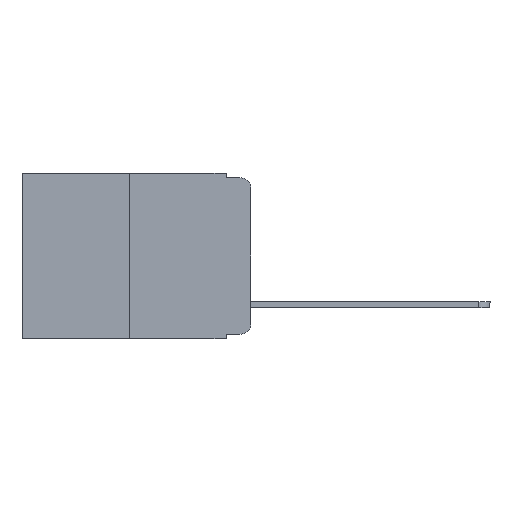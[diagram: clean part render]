
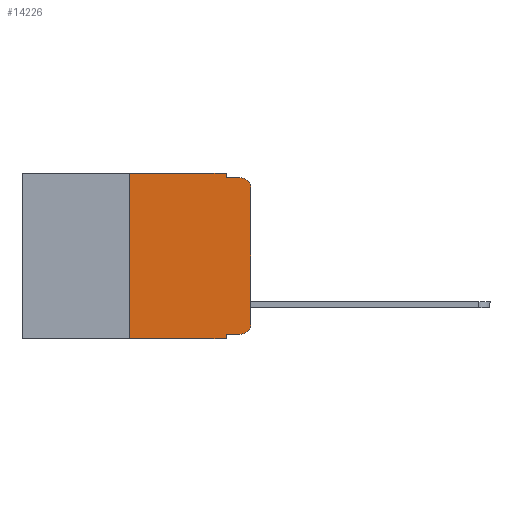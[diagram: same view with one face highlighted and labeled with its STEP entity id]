
A CAD part, left-side view. The second image highlights one B-rep face of the part: STEP entity #14226.
In plain terms, the highlighted planar face has unit normal (-1, 0, 0).
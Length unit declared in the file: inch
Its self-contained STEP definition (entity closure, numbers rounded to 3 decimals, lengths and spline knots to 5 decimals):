
#185 = DIRECTION ( 'NONE',  ( -1., 0., 0. ) ) ;
#280 = LINE ( 'NONE', #7466, #1851 ) ;
#344 = EDGE_CURVE ( 'NONE', #2409, #5183, #1535, .T. ) ;
#446 = VERTEX_POINT ( 'NONE', #1766 ) ;
#657 = DIRECTION ( 'NONE',  ( 0., -1., 0. ) ) ;
#705 = CARTESIAN_POINT ( 'NONE',  ( 0., 0.051, -0.01 ) ) ;
#978 = VECTOR ( 'NONE', #13768, 39.37008 ) ;
#1535 = LINE ( 'NONE', #14655, #6541 ) ;
#1602 = ORIENTED_EDGE ( 'NONE', *, *, #10612, .T. ) ;
#1671 = CARTESIAN_POINT ( 'NONE',  ( 0., 0., 0. ) ) ;
#1766 = CARTESIAN_POINT ( 'NONE',  ( 0., 0.25, -0.343 ) ) ;
#1851 = VECTOR ( 'NONE', #11121, 39.37008 ) ;
#1924 = DIRECTION ( 'NONE',  ( 0., 0., -1. ) ) ;
#1934 = VECTOR ( 'NONE', #12758, 39.37008 ) ;
#1949 = CARTESIAN_POINT ( 'NONE',  ( 0., 0., -0.03 ) ) ;
#2409 = VERTEX_POINT ( 'NONE', #8047 ) ;
#2477 = VECTOR ( 'NONE', #13080, 39.37008 ) ;
#2598 = CARTESIAN_POINT ( 'NONE',  ( 0., 0.02, -0.333 ) ) ;
#2870 = CARTESIAN_POINT ( 'NONE',  ( 0., 0.02, -0.01 ) ) ;
#3185 = ORIENTED_EDGE ( 'NONE', *, *, #9227, .F. ) ;
#3353 = LINE ( 'NONE', #7112, #5580 ) ;
#3398 = FACE_OUTER_BOUND ( 'NONE', #4517, .T. ) ;
#3607 = EDGE_CURVE ( 'NONE', #5183, #8380, #280, .T. ) ;
#3684 = ORIENTED_EDGE ( 'NONE', *, *, #11740, .F. ) ;
#3783 = EDGE_CURVE ( 'NONE', #3950, #15179, #3353, .T. ) ;
#3950 = VERTEX_POINT ( 'NONE', #9842 ) ;
#4175 = CARTESIAN_POINT ( 'NONE',  ( 0., 0.02, -0.313 ) ) ;
#4394 = DIRECTION ( 'NONE',  ( 0., -1., 0. ) ) ;
#4517 = EDGE_LOOP ( 'NONE', ( #15356, #11293, #3684, #7398, #9274, #3185, #8095, #13039, #12445, #1602 ) ) ;
#4540 = VERTEX_POINT ( 'NONE', #2870 ) ;
#5015 = CARTESIAN_POINT ( 'NONE',  ( 0., 0., -0.313 ) ) ;
#5183 = VERTEX_POINT ( 'NONE', #9634 ) ;
#5199 = LINE ( 'NONE', #14750, #12149 ) ;
#5580 = VECTOR ( 'NONE', #14138, 39.37008 ) ;
#5944 = AXIS2_PLACEMENT_3D ( 'NONE', #4175, #6682, #1924 ) ;
#6128 = CARTESIAN_POINT ( 'NONE',  ( 0., 0.051, 0. ) ) ;
#6350 = VERTEX_POINT ( 'NONE', #5015 ) ;
#6395 = EDGE_CURVE ( 'NONE', #7054, #4540, #9775, .T. ) ;
#6521 = CARTESIAN_POINT ( 'NONE',  ( 0., 0.25, 0. ) ) ;
#6541 = VECTOR ( 'NONE', #4394, 39.37008 ) ;
#6588 = LINE ( 'NONE', #11349, #14946 ) ;
#6682 = DIRECTION ( 'NONE',  ( -1., 0., 0. ) ) ;
#6790 = AXIS2_PLACEMENT_3D ( 'NONE', #8303, #185, #14241 ) ;
#7054 = VERTEX_POINT ( 'NONE', #1949 ) ;
#7112 = CARTESIAN_POINT ( 'NONE',  ( 0., 0.051, -0.333 ) ) ;
#7398 = ORIENTED_EDGE ( 'NONE', *, *, #3607, .F. ) ;
#7466 = CARTESIAN_POINT ( 'NONE',  ( 0., 0.051, 0. ) ) ;
#8002 = LINE ( 'NONE', #6521, #1934 ) ;
#8047 = CARTESIAN_POINT ( 'NONE',  ( 0., 0.25, 0. ) ) ;
#8095 = ORIENTED_EDGE ( 'NONE', *, *, #11150, .T. ) ;
#8303 = CARTESIAN_POINT ( 'NONE',  ( 0., 0.02, -0.03 ) ) ;
#8380 = VERTEX_POINT ( 'NONE', #705 ) ;
#8397 = LINE ( 'NONE', #6128, #2477 ) ;
#8643 = CARTESIAN_POINT ( 'NONE',  ( 0., 0.051, -0.343 ) ) ;
#9007 = LINE ( 'NONE', #1671, #978 ) ;
#9227 = EDGE_CURVE ( 'NONE', #446, #2409, #8002, .T. ) ;
#9274 = ORIENTED_EDGE ( 'NONE', *, *, #344, .F. ) ;
#9634 = CARTESIAN_POINT ( 'NONE',  ( 0., 0.051, 0. ) ) ;
#9775 = CIRCLE ( 'NONE', #6790, 0.02 ) ;
#9819 = DIRECTION ( 'NONE',  ( 0., -1., 0. ) ) ;
#9842 = CARTESIAN_POINT ( 'NONE',  ( 0., 0.051, -0.333 ) ) ;
#10612 = EDGE_CURVE ( 'NONE', #15179, #6350, #12690, .T. ) ;
#10751 = DIRECTION ( 'NONE',  ( 0., 0., -1. ) ) ;
#10968 = EDGE_CURVE ( 'NONE', #3950, #14391, #8397, .T. ) ;
#11121 = DIRECTION ( 'NONE',  ( 0., 0., -1. ) ) ;
#11150 = EDGE_CURVE ( 'NONE', #446, #14391, #6588, .T. ) ;
#11293 = ORIENTED_EDGE ( 'NONE', *, *, #6395, .T. ) ;
#11349 = CARTESIAN_POINT ( 'NONE',  ( 0., 0.473, -0.343 ) ) ;
#11472 = AXIS2_PLACEMENT_3D ( 'NONE', #12934, #13011, #10751 ) ;
#11680 = PLANE ( 'NONE',  #11472 ) ;
#11740 = EDGE_CURVE ( 'NONE', #8380, #4540, #5199, .T. ) ;
#12149 = VECTOR ( 'NONE', #9819, 39.37008 ) ;
#12445 = ORIENTED_EDGE ( 'NONE', *, *, #3783, .T. ) ;
#12690 = CIRCLE ( 'NONE', #5944, 0.02 ) ;
#12758 = DIRECTION ( 'NONE',  ( 0., 0., 1. ) ) ;
#12934 = CARTESIAN_POINT ( 'NONE',  ( 0., 0.473, 0. ) ) ;
#13011 = DIRECTION ( 'NONE',  ( 1., 0., 0. ) ) ;
#13039 = ORIENTED_EDGE ( 'NONE', *, *, #10968, .F. ) ;
#13080 = DIRECTION ( 'NONE',  ( 0., 0., -1. ) ) ;
#13658 = EDGE_CURVE ( 'NONE', #6350, #7054, #9007, .T. ) ;
#13768 = DIRECTION ( 'NONE',  ( 0., 0., 1. ) ) ;
#14138 = DIRECTION ( 'NONE',  ( 0., -1., 0. ) ) ;
#14226 = ADVANCED_FACE ( 'NONE', ( #3398 ), #11680, .F. ) ;
#14241 = DIRECTION ( 'NONE',  ( 0., 0., -1. ) ) ;
#14391 = VERTEX_POINT ( 'NONE', #8643 ) ;
#14655 = CARTESIAN_POINT ( 'NONE',  ( 0., 0.473, 0. ) ) ;
#14750 = CARTESIAN_POINT ( 'NONE',  ( 0., 0.051, -0.01 ) ) ;
#14946 = VECTOR ( 'NONE', #657, 39.37008 ) ;
#15179 = VERTEX_POINT ( 'NONE', #2598 ) ;
#15356 = ORIENTED_EDGE ( 'NONE', *, *, #13658, .T. ) ;
